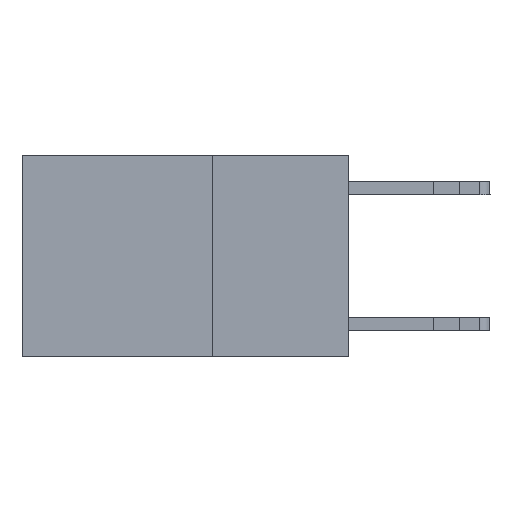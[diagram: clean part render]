
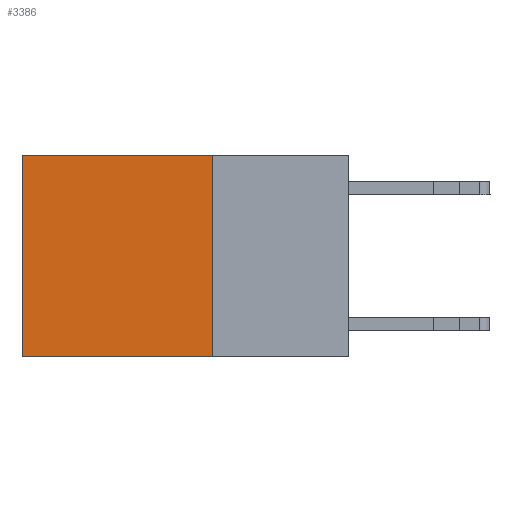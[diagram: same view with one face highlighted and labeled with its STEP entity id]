
A CAD part, left-side view. The second image highlights one B-rep face of the part: STEP entity #3386.
In plain terms, the highlighted planar face has unit normal (-1, 0, 0).
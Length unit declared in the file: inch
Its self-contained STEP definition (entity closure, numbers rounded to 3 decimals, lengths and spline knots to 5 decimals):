
#440 = CARTESIAN_POINT ( 'NONE',  ( 0.2625, 0.25, -0.37 ) ) ;
#650 = LINE ( 'NONE', #9494, #3520 ) ;
#1160 = CARTESIAN_POINT ( 'NONE',  ( 0.2625, 0.6, 0. ) ) ;
#2444 = DIRECTION ( 'NONE',  ( 0., 0., -1. ) ) ;
#2836 = VERTEX_POINT ( 'NONE', #440 ) ;
#2926 = CARTESIAN_POINT ( 'NONE',  ( 0.2625, 0.25, 0. ) ) ;
#3386 = ADVANCED_FACE ( 'NONE', ( #5061 ), #6807, .F. ) ;
#3520 = VECTOR ( 'NONE', #12526, 39.37008 ) ;
#3669 = DIRECTION ( 'NONE',  ( 0., 1., 0. ) ) ;
#4057 = DIRECTION ( 'NONE',  ( 0., 1., 0. ) ) ;
#4487 = EDGE_CURVE ( 'NONE', #11822, #11197, #8044, .T. ) ;
#4625 = EDGE_CURVE ( 'NONE', #11197, #11601, #650, .T. ) ;
#5061 = FACE_OUTER_BOUND ( 'NONE', #11987, .T. ) ;
#5201 = VECTOR ( 'NONE', #4057, 39.37008 ) ;
#5759 = EDGE_CURVE ( 'NONE', #11822, #2836, #8177, .T. ) ;
#6016 = ORIENTED_EDGE ( 'NONE', *, *, #6972, .F. ) ;
#6807 = PLANE ( 'NONE',  #13186 ) ;
#6972 = EDGE_CURVE ( 'NONE', #2836, #11601, #10058, .T. ) ;
#7634 = VECTOR ( 'NONE', #3669, 39.37008 ) ;
#7853 = CARTESIAN_POINT ( 'NONE',  ( 0.2625, 0.25, 0. ) ) ;
#8044 = LINE ( 'NONE', #2926, #5201 ) ;
#8177 = LINE ( 'NONE', #11105, #13534 ) ;
#8462 = ORIENTED_EDGE ( 'NONE', *, *, #4625, .T. ) ;
#8794 = ORIENTED_EDGE ( 'NONE', *, *, #5759, .F. ) ;
#8905 = DIRECTION ( 'NONE',  ( 1., 0., 0. ) ) ;
#8966 = CARTESIAN_POINT ( 'NONE',  ( 0.2625, 0.25, -0.37 ) ) ;
#9120 = ORIENTED_EDGE ( 'NONE', *, *, #4487, .T. ) ;
#9494 = CARTESIAN_POINT ( 'NONE',  ( 0.2625, 0.6, 0. ) ) ;
#10058 = LINE ( 'NONE', #8966, #7634 ) ;
#11105 = CARTESIAN_POINT ( 'NONE',  ( 0.2625, 0.25, 0. ) ) ;
#11197 = VERTEX_POINT ( 'NONE', #1160 ) ;
#11307 = CARTESIAN_POINT ( 'NONE',  ( 0.2625, 0.6, -0.37 ) ) ;
#11601 = VERTEX_POINT ( 'NONE', #11307 ) ;
#11822 = VERTEX_POINT ( 'NONE', #12483 ) ;
#11987 = EDGE_LOOP ( 'NONE', ( #8462, #6016, #8794, #9120 ) ) ;
#12114 = DIRECTION ( 'NONE',  ( 0., 0., -1. ) ) ;
#12483 = CARTESIAN_POINT ( 'NONE',  ( 0.2625, 0.25, 0. ) ) ;
#12526 = DIRECTION ( 'NONE',  ( 0., 0., -1. ) ) ;
#13186 = AXIS2_PLACEMENT_3D ( 'NONE', #7853, #8905, #2444 ) ;
#13534 = VECTOR ( 'NONE', #12114, 39.37008 ) ;
